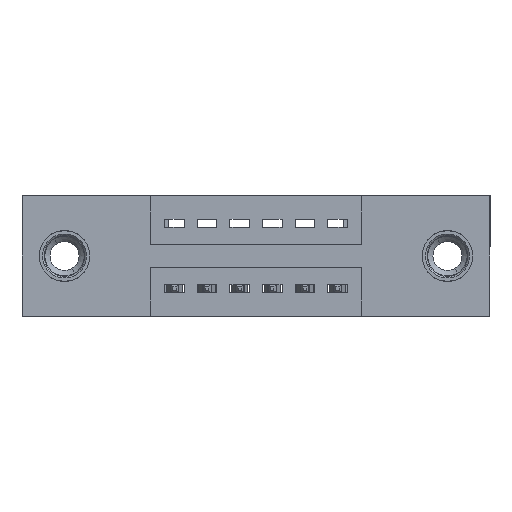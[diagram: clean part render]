
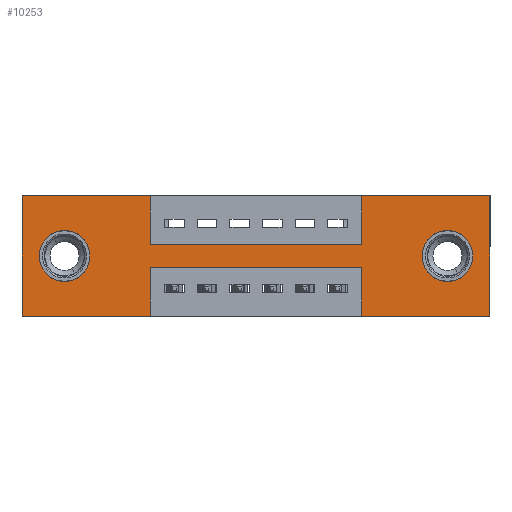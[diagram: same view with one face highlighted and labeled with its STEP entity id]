
A CAD part, front view. The second image highlights one B-rep face of the part: STEP entity #10253.
In plain terms, the highlighted planar face has unit normal (0, -1, 0).
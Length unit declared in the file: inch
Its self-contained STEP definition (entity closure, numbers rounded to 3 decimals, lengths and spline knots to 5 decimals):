
#39 = DIRECTION ( 'NONE',  ( 0., 0., 1. ) ) ;
#127 = CARTESIAN_POINT ( 'NONE',  ( 1.0425, 0., 0. ) ) ;
#392 = DIRECTION ( 'NONE',  ( 0., 0., -1. ) ) ;
#418 = CARTESIAN_POINT ( 'NONE',  ( 1.0425, 0., -0.37 ) ) ;
#521 = FACE_OUTER_BOUND ( 'NONE', #10496, .T. ) ;
#579 = EDGE_CURVE ( 'NONE', #11269, #7327, #10247, .T. ) ;
#667 = LINE ( 'NONE', #2101, #1787 ) ;
#870 = VERTEX_POINT ( 'NONE', #10572 ) ;
#912 = CARTESIAN_POINT ( 'NONE',  ( 1.0425, 0., -0.37 ) ) ;
#1138 = CARTESIAN_POINT ( 'NONE',  ( 0.3925, 0., 0. ) ) ;
#1244 = CIRCLE ( 'NONE', #8079, 0.078 ) ;
#1473 = DIRECTION ( 'NONE',  ( 1., 0., 0. ) ) ;
#1529 = DIRECTION ( 'NONE',  ( 0., -1., 0. ) ) ;
#1622 = VERTEX_POINT ( 'NONE', #418 ) ;
#1658 = CARTESIAN_POINT ( 'NONE',  ( 1.305, 0., -0.185 ) ) ;
#1684 = DIRECTION ( 'NONE',  ( 0., 1., 0. ) ) ;
#1739 = DIRECTION ( 'NONE',  ( 0., 0., 1. ) ) ;
#1787 = VECTOR ( 'NONE', #6663, 39.37008 ) ;
#1810 = DIRECTION ( 'NONE',  ( -1., 0., 0. ) ) ;
#1876 = DIRECTION ( 'NONE',  ( 1., 0., 0. ) ) ;
#1915 = EDGE_CURVE ( 'NONE', #4896, #3049, #1983, .T. ) ;
#1983 = LINE ( 'NONE', #8907, #5717 ) ;
#2101 = CARTESIAN_POINT ( 'NONE',  ( 0.3925, 0., 0. ) ) ;
#2169 = VERTEX_POINT ( 'NONE', #3046 ) ;
#2268 = VERTEX_POINT ( 'NONE', #9407 ) ;
#2275 = CIRCLE ( 'NONE', #3903, 0.078 ) ;
#2286 = EDGE_CURVE ( 'NONE', #5165, #870, #6006, .T. ) ;
#2297 = ORIENTED_EDGE ( 'NONE', *, *, #7195, .F. ) ;
#2303 = CARTESIAN_POINT ( 'NONE',  ( 0.3925, 0., -0.15 ) ) ;
#2330 = DIRECTION ( 'NONE',  ( 0., 0., 1. ) ) ;
#2517 = VERTEX_POINT ( 'NONE', #7480 ) ;
#2646 = LINE ( 'NONE', #4396, #6426 ) ;
#2815 = CARTESIAN_POINT ( 'NONE',  ( 0.13, 0., -0.263 ) ) ;
#2819 = EDGE_CURVE ( 'NONE', #1622, #5165, #8787, .T. ) ;
#2832 = CARTESIAN_POINT ( 'NONE',  ( 0.13, 0., -0.185 ) ) ;
#2852 = ORIENTED_EDGE ( 'NONE', *, *, #6520, .T. ) ;
#2947 = EDGE_CURVE ( 'NONE', #2169, #1622, #2646, .T. ) ;
#2962 = VECTOR ( 'NONE', #1876, 39.37008 ) ;
#3028 = CARTESIAN_POINT ( 'NONE',  ( 1.0425, 0., -0.22 ) ) ;
#3046 = CARTESIAN_POINT ( 'NONE',  ( 1.435, 0., -0.37 ) ) ;
#3049 = VERTEX_POINT ( 'NONE', #10878 ) ;
#3089 = EDGE_CURVE ( 'NONE', #2517, #7231, #1244, .T. ) ;
#3168 = VERTEX_POINT ( 'NONE', #7028 ) ;
#3198 = CARTESIAN_POINT ( 'NONE',  ( 0., 0., 0. ) ) ;
#3367 = VECTOR ( 'NONE', #1473, 39.37008 ) ;
#3435 = VERTEX_POINT ( 'NONE', #1138 ) ;
#3438 = VECTOR ( 'NONE', #10238, 39.37008 ) ;
#3548 = CARTESIAN_POINT ( 'NONE',  ( 1.0425, 0., 0. ) ) ;
#3619 = VECTOR ( 'NONE', #11106, 39.37008 ) ;
#3631 = VECTOR ( 'NONE', #8591, 39.37008 ) ;
#3903 = AXIS2_PLACEMENT_3D ( 'NONE', #2832, #9056, #8392 ) ;
#3913 = CARTESIAN_POINT ( 'NONE',  ( 0., 0., -0.37 ) ) ;
#4006 = AXIS2_PLACEMENT_3D ( 'NONE', #9716, #1529, #9677 ) ;
#4010 = ORIENTED_EDGE ( 'NONE', *, *, #6451, .F. ) ;
#4170 = ORIENTED_EDGE ( 'NONE', *, *, #8189, .F. ) ;
#4174 = LINE ( 'NONE', #5637, #3619 ) ;
#4198 = ORIENTED_EDGE ( 'NONE', *, *, #2286, .F. ) ;
#4215 = EDGE_CURVE ( 'NONE', #3435, #3168, #667, .T. ) ;
#4265 = EDGE_CURVE ( 'NONE', #2268, #8164, #5527, .T. ) ;
#4302 = CARTESIAN_POINT ( 'NONE',  ( 0.3925, 0., -0.37 ) ) ;
#4317 = DIRECTION ( 'NONE',  ( 0., 0., -1. ) ) ;
#4396 = CARTESIAN_POINT ( 'NONE',  ( 0., 0., -0.37 ) ) ;
#4397 = CARTESIAN_POINT ( 'NONE',  ( 1.0425, 0., -0.15 ) ) ;
#4401 = FACE_BOUND ( 'NONE', #9531, .T. ) ;
#4738 = CARTESIAN_POINT ( 'NONE',  ( 1.435, 0., 0. ) ) ;
#4771 = VECTOR ( 'NONE', #5777, 39.37008 ) ;
#4896 = VERTEX_POINT ( 'NONE', #9798 ) ;
#5149 = ORIENTED_EDGE ( 'NONE', *, *, #4215, .F. ) ;
#5165 = VERTEX_POINT ( 'NONE', #3028 ) ;
#5342 = DIRECTION ( 'NONE',  ( 0., 0., 1. ) ) ;
#5527 = CIRCLE ( 'NONE', #10244, 0.078 ) ;
#5606 = EDGE_LOOP ( 'NONE', ( #6329, #9100 ) ) ;
#5637 = CARTESIAN_POINT ( 'NONE',  ( 0.3925, 0., -0.37 ) ) ;
#5717 = VECTOR ( 'NONE', #39, 39.37008 ) ;
#5777 = DIRECTION ( 'NONE',  ( -1., 0., 0. ) ) ;
#5804 = LINE ( 'NONE', #3198, #3438 ) ;
#5899 = LINE ( 'NONE', #3913, #4771 ) ;
#5982 = EDGE_CURVE ( 'NONE', #9166, #4896, #5899, .T. ) ;
#5997 = PLANE ( 'NONE',  #4006 ) ;
#6006 = LINE ( 'NONE', #8839, #3631 ) ;
#6122 = CARTESIAN_POINT ( 'NONE',  ( 1.305, 0., -0.107 ) ) ;
#6329 = ORIENTED_EDGE ( 'NONE', *, *, #7229, .T. ) ;
#6426 = VECTOR ( 'NONE', #1810, 39.37008 ) ;
#6451 = EDGE_CURVE ( 'NONE', #3049, #3435, #10927, .T. ) ;
#6520 = EDGE_CURVE ( 'NONE', #8164, #2268, #2275, .T. ) ;
#6610 = EDGE_CURVE ( 'NONE', #3168, #11269, #6735, .T. ) ;
#6663 = DIRECTION ( 'NONE',  ( 0., 0., -1. ) ) ;
#6735 = LINE ( 'NONE', #2303, #3367 ) ;
#7028 = CARTESIAN_POINT ( 'NONE',  ( 0.3925, 0., -0.15 ) ) ;
#7195 = EDGE_CURVE ( 'NONE', #10528, #2169, #10080, .T. ) ;
#7229 = EDGE_CURVE ( 'NONE', #7231, #2517, #7280, .T. ) ;
#7231 = VERTEX_POINT ( 'NONE', #6122 ) ;
#7238 = CARTESIAN_POINT ( 'NONE',  ( 0., 0., 0. ) ) ;
#7262 = ORIENTED_EDGE ( 'NONE', *, *, #5982, .F. ) ;
#7280 = CIRCLE ( 'NONE', #8542, 0.078 ) ;
#7327 = VERTEX_POINT ( 'NONE', #127 ) ;
#7445 = VECTOR ( 'NONE', #5342, 39.37008 ) ;
#7480 = CARTESIAN_POINT ( 'NONE',  ( 1.305, 0., -0.263 ) ) ;
#7687 = DIRECTION ( 'NONE',  ( 0., 1., 0. ) ) ;
#7763 = ORIENTED_EDGE ( 'NONE', *, *, #4265, .T. ) ;
#8035 = DIRECTION ( 'NONE',  ( 0., 0., -1. ) ) ;
#8079 = AXIS2_PLACEMENT_3D ( 'NONE', #8754, #1684, #8035 ) ;
#8164 = VERTEX_POINT ( 'NONE', #2815 ) ;
#8189 = EDGE_CURVE ( 'NONE', #870, #9166, #4174, .T. ) ;
#8392 = DIRECTION ( 'NONE',  ( 0., 0., 1. ) ) ;
#8526 = ORIENTED_EDGE ( 'NONE', *, *, #9586, .F. ) ;
#8542 = AXIS2_PLACEMENT_3D ( 'NONE', #1658, #8814, #4317 ) ;
#8591 = DIRECTION ( 'NONE',  ( -1., 0., 0. ) ) ;
#8754 = CARTESIAN_POINT ( 'NONE',  ( 1.305, 0., -0.185 ) ) ;
#8787 = LINE ( 'NONE', #912, #10047 ) ;
#8793 = ORIENTED_EDGE ( 'NONE', *, *, #2947, .F. ) ;
#8814 = DIRECTION ( 'NONE',  ( 0., 1., 0. ) ) ;
#8839 = CARTESIAN_POINT ( 'NONE',  ( 0.3925, 0., -0.22 ) ) ;
#8907 = CARTESIAN_POINT ( 'NONE',  ( 0., 0., 0. ) ) ;
#9056 = DIRECTION ( 'NONE',  ( 0., 1., 0. ) ) ;
#9100 = ORIENTED_EDGE ( 'NONE', *, *, #3089, .T. ) ;
#9144 = FACE_BOUND ( 'NONE', #5606, .T. ) ;
#9166 = VERTEX_POINT ( 'NONE', #4302 ) ;
#9311 = ORIENTED_EDGE ( 'NONE', *, *, #579, .F. ) ;
#9351 = VECTOR ( 'NONE', #392, 39.37008 ) ;
#9407 = CARTESIAN_POINT ( 'NONE',  ( 0.13, 0., -0.107 ) ) ;
#9531 = EDGE_LOOP ( 'NONE', ( #7763, #2852 ) ) ;
#9586 = EDGE_CURVE ( 'NONE', #7327, #10528, #5804, .T. ) ;
#9677 = DIRECTION ( 'NONE',  ( 0., 0., -1. ) ) ;
#9716 = CARTESIAN_POINT ( 'NONE',  ( 0., 0., -0.37 ) ) ;
#9798 = CARTESIAN_POINT ( 'NONE',  ( 0., 0., -0.37 ) ) ;
#9927 = ORIENTED_EDGE ( 'NONE', *, *, #1915, .F. ) ;
#10019 = ORIENTED_EDGE ( 'NONE', *, *, #2819, .F. ) ;
#10047 = VECTOR ( 'NONE', #1739, 39.37008 ) ;
#10080 = LINE ( 'NONE', #4738, #9351 ) ;
#10238 = DIRECTION ( 'NONE',  ( 1., 0., 0. ) ) ;
#10244 = AXIS2_PLACEMENT_3D ( 'NONE', #10413, #7687, #2330 ) ;
#10247 = LINE ( 'NONE', #3548, #7445 ) ;
#10253 = ADVANCED_FACE ( 'NONE', ( #9144, #4401, #521 ), #5997, .T. ) ;
#10413 = CARTESIAN_POINT ( 'NONE',  ( 0.13, 0., -0.185 ) ) ;
#10496 = EDGE_LOOP ( 'NONE', ( #4170, #4198, #10019, #8793, #2297, #8526, #9311, #11080, #5149, #4010, #9927, #7262 ) ) ;
#10528 = VERTEX_POINT ( 'NONE', #10974 ) ;
#10572 = CARTESIAN_POINT ( 'NONE',  ( 0.3925, 0., -0.22 ) ) ;
#10878 = CARTESIAN_POINT ( 'NONE',  ( 0., 0., 0. ) ) ;
#10927 = LINE ( 'NONE', #7238, #2962 ) ;
#10974 = CARTESIAN_POINT ( 'NONE',  ( 1.435, 0., 0. ) ) ;
#11080 = ORIENTED_EDGE ( 'NONE', *, *, #6610, .F. ) ;
#11106 = DIRECTION ( 'NONE',  ( 0., 0., -1. ) ) ;
#11269 = VERTEX_POINT ( 'NONE', #4397 ) ;
